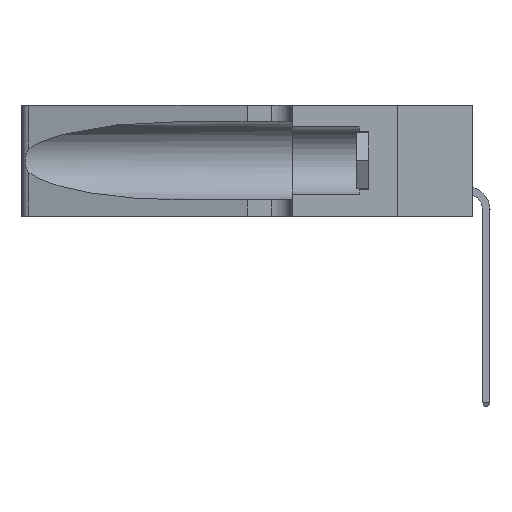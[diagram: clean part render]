
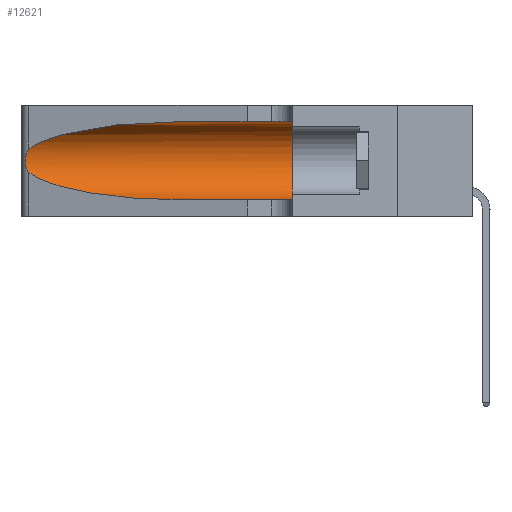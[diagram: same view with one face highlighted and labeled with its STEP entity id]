
A CAD part, left-side view. The second image highlights one B-rep face of the part: STEP entity #12621.
In plain terms, the highlighted cylindrical face has radius 3.308 mm (diameter 6.617 mm), a partial arc.
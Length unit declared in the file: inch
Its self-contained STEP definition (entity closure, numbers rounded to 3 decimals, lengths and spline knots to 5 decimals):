
#13 = CARTESIAN_POINT ( 'NONE',  ( 0.1305, 0.35, 0.31525 ) ) ;
#126 = LINE ( 'NONE', #25680, #47708 ) ;
#1522 = VERTEX_POINT ( 'NONE', #13 ) ;
#2259 = EDGE_CURVE ( 'NONE', #1522, #35815, #10833, .T. ) ;
#2739 = CARTESIAN_POINT ( 'NONE',  ( 0.18966, 0.96281, 0.05475 ) ) ;
#5350 = VERTEX_POINT ( 'NONE', #44495 ) ;
#6171 = AXIS2_PLACEMENT_3D ( 'NONE', #7234, #17791, #33782 ) ;
#6755 = CARTESIAN_POINT ( 'NONE',  ( 0.25555, 1.22993, 0.14849 ) ) ;
#7234 = CARTESIAN_POINT ( 'NONE',  ( 0.1305, 0.35, 0.185 ) ) ;
#8031 = EDGE_CURVE ( 'NONE', #14343, #5350, #34232, .T. ) ;
#8423 = ORIENTED_EDGE ( 'NONE', *, *, #2259, .F. ) ;
#9697 = CARTESIAN_POINT ( 'NONE',  ( 0.25787, 1.23484, 0.2124 ) ) ;
#10833 = CIRCLE ( 'NONE', #6171, 0.13025 ) ;
#11601 = ORIENTED_EDGE ( 'NONE', *, *, #25747, .T. ) ;
#12621 = ADVANCED_FACE ( 'NONE', ( #45623 ), #19786, .F. ) ;
#13343 = CARTESIAN_POINT ( 'NONE',  ( 0.25487, 1.22718, 0.22369 ) ) ;
#13512 = CARTESIAN_POINT ( 'NONE',  ( 0.25854, 1.2359, 0.20912 ) ) ;
#13620 = VECTOR ( 'NONE', #37139, 39.37008 ) ;
#14343 = VERTEX_POINT ( 'NONE', #42502 ) ;
#14344 = CARTESIAN_POINT ( 'NONE',  ( 0.26075, 1.23896, 0.19203 ) ) ;
#16061 = CARTESIAN_POINT ( 'NONE',  ( 0.2373, 1.15595, 0.28018 ) ) ;
#16508 = EDGE_CURVE ( 'NONE', #24609, #1522, #44120, .T. ) ;
#16884 = ORIENTED_EDGE ( 'NONE', *, *, #28162, .T. ) ;
#17278 = CARTESIAN_POINT ( 'NONE',  ( 0.26075, 1.23896, 0.178 ) ) ;
#17710 = CARTESIAN_POINT ( 'NONE',  ( 0.1305, 0.72297, 0.05475 ) ) ;
#17791 = DIRECTION ( 'NONE',  ( 0., 1., 0. ) ) ;
#18831 = DIRECTION ( 'NONE',  ( 0., -1., 0. ) ) ;
#19786 = CYLINDRICAL_SURFACE ( 'NONE', #21653, 0.13025 ) ;
#20936 = CARTESIAN_POINT ( 'NONE',  ( 0.25555, 1.22994, 0.2215 ) ) ;
#21653 = AXIS2_PLACEMENT_3D ( 'NONE', #48410, #18831, #25920 ) ;
#21655 = CARTESIAN_POINT ( 'NONE',  ( 0.1305, 1.61858, 0.31525 ) ) ;
#24111 = CARTESIAN_POINT ( 'NONE',  ( 0.25487, 1.22718, 0.22369 ) ) ;
#24609 = VERTEX_POINT ( 'NONE', #38349 ) ;
#24810 = CARTESIAN_POINT ( 'NONE',  ( 0.25789, 1.23486, 0.15765 ) ) ;
#25576 = CARTESIAN_POINT ( 'NONE',  ( 0.2373, 1.15595, 0.08982 ) ) ;
#25680 = CARTESIAN_POINT ( 'NONE',  ( 0.1305, 1.61858, 0.05475 ) ) ;
#25747 = EDGE_CURVE ( 'NONE', #24609, #14343, #40003, .T. ) ;
#25920 = DIRECTION ( 'NONE',  ( 0., 0., -1. ) ) ;
#28162 = EDGE_CURVE ( 'NONE', #5350, #35867, #42354, .T. ) ;
#29250 = CARTESIAN_POINT ( 'NONE',  ( 0.25639, 1.23186, 0.15144 ) ) ;
#29889 = DIRECTION ( 'NONE',  ( 0., -1., 0. ) ) ;
#31077 = CARTESIAN_POINT ( 'NONE',  ( 0.1305, 0.72297, 0.31525 ) ) ;
#32164 = CARTESIAN_POINT ( 'NONE',  ( 0.25639, 1.23184, 0.21858 ) ) ;
#33012 = CARTESIAN_POINT ( 'NONE',  ( 0.25487, 1.22718, 0.14631 ) ) ;
#33782 = DIRECTION ( 'NONE',  ( 0., 0., 1. ) ) ;
#34232 = B_SPLINE_CURVE_WITH_KNOTS ( 'NONE', 3,
 ( #13343, #20936, #32164, #9697, #13512, #35942, #14344, #17278, #39712, #47308, #24810, #29250, #6755, #33012 ),
 .UNSPECIFIED., .F., .F.,
 ( 4, 2, 2, 2, 2, 2, 4 ),
 ( 0., 0.00027, 0.00053, 0.00107, 0.0016, 0.00187, 0.00214 ),
 .UNSPECIFIED. ) ;
#35227 = ORIENTED_EDGE ( 'NONE', *, *, #8031, .T. ) ;
#35232 = CARTESIAN_POINT ( 'NONE',  ( 0.18966, 0.96281, 0.31525 ) ) ;
#35440 = CARTESIAN_POINT ( 'NONE',  ( 0.1305, 0.35, 0.05475 ) ) ;
#35815 = VERTEX_POINT ( 'NONE', #35440 ) ;
#35867 = VERTEX_POINT ( 'NONE', #47511 ) ;
#35942 = CARTESIAN_POINT ( 'NONE',  ( 0.26018, 1.23835, 0.19895 ) ) ;
#36218 = CARTESIAN_POINT ( 'NONE',  ( 0.25487, 1.22718, 0.14631 ) ) ;
#37103 = EDGE_CURVE ( 'NONE', #35867, #35815, #126, .T. ) ;
#37139 = DIRECTION ( 'NONE',  ( 0., -1., 0. ) ) ;
#38059 = ORIENTED_EDGE ( 'NONE', *, *, #37103, .T. ) ;
#38349 = CARTESIAN_POINT ( 'NONE',  ( 0.1305, 0.72297, 0.31525 ) ) ;
#39712 = CARTESIAN_POINT ( 'NONE',  ( 0.26017, 1.23833, 0.17102 ) ) ;
#40003 =( BOUNDED_CURVE ( )  B_SPLINE_CURVE ( 3, ( #31077, #35232, #16061, #24111 ),
 .UNSPECIFIED., .F., .F. ) 
 B_SPLINE_CURVE_WITH_KNOTS ( ( 4, 4 ),
 ( 1.5708, 2.84003 ),
 .UNSPECIFIED. ) 
 CURVE ( )  GEOMETRIC_REPRESENTATION_ITEM ( )  RATIONAL_B_SPLINE_CURVE ( ( 1., 0.87, 0.87, 1. ) ) 
 REPRESENTATION_ITEM ( '' )  );
#42354 =( BOUNDED_CURVE ( )  B_SPLINE_CURVE ( 3, ( #36218, #25576, #2739, #17710 ),
 .UNSPECIFIED., .F., .F. ) 
 B_SPLINE_CURVE_WITH_KNOTS ( ( 4, 4 ),
 ( 3.44316, 4.71239 ),
 .UNSPECIFIED. ) 
 CURVE ( )  GEOMETRIC_REPRESENTATION_ITEM ( )  RATIONAL_B_SPLINE_CURVE ( ( 1., 0.87, 0.87, 1. ) ) 
 REPRESENTATION_ITEM ( '' )  );
#42502 = CARTESIAN_POINT ( 'NONE',  ( 0.25487, 1.22718, 0.22369 ) ) ;
#44120 = LINE ( 'NONE', #21655, #13620 ) ;
#44495 = CARTESIAN_POINT ( 'NONE',  ( 0.25487, 1.22718, 0.14631 ) ) ;
#45623 = FACE_OUTER_BOUND ( 'NONE', #46012, .T. ) ;
#46012 = EDGE_LOOP ( 'NONE', ( #11601, #35227, #16884, #38059, #8423, #48439 ) ) ;
#47308 = CARTESIAN_POINT ( 'NONE',  ( 0.25856, 1.23593, 0.16098 ) ) ;
#47511 = CARTESIAN_POINT ( 'NONE',  ( 0.1305, 0.72297, 0.05475 ) ) ;
#47708 = VECTOR ( 'NONE', #29889, 39.37008 ) ;
#48410 = CARTESIAN_POINT ( 'NONE',  ( 0.1305, 1.61858, 0.185 ) ) ;
#48439 = ORIENTED_EDGE ( 'NONE', *, *, #16508, .F. ) ;
